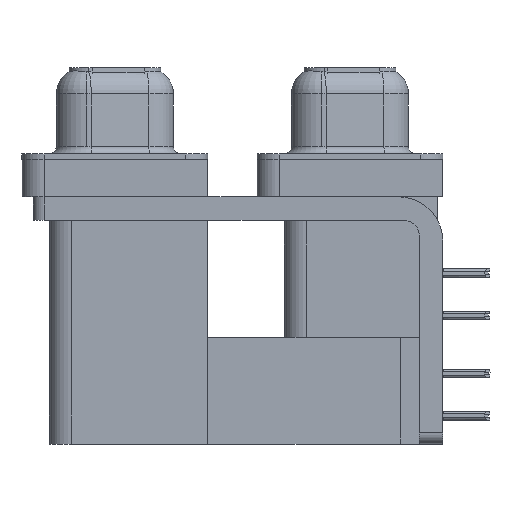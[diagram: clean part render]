
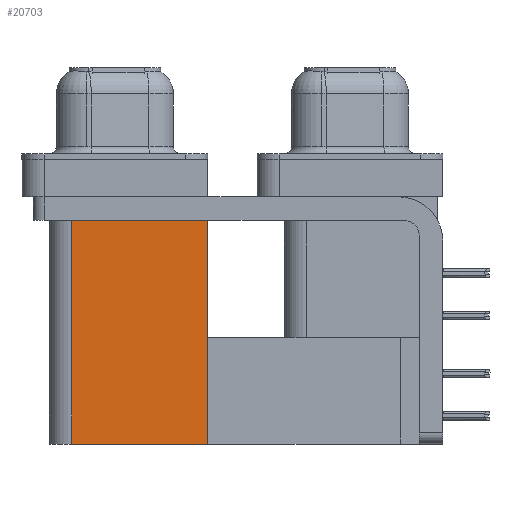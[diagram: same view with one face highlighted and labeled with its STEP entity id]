
A CAD part, left-side view. The second image highlights one B-rep face of the part: STEP entity #20703.
In plain terms, the highlighted planar face has unit normal (-1, 0, 0).
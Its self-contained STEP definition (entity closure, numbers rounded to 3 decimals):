
#414 = EDGE_LOOP ( 'NONE', ( #9006, #5287, #41787, #28909 ) ) ;
#511 = DIRECTION ( 'NONE',  ( 1., 0., 0. ) ) ;
#982 = CARTESIAN_POINT ( 'NONE',  ( 3.765, 9.6, -19.2 ) ) ;
#1129 = CARTESIAN_POINT ( 'NONE',  ( 3.765, 18.8, -19.2 ) ) ;
#2963 = CARTESIAN_POINT ( 'NONE',  ( 3.765, 18.8, -2.5 ) ) ;
#3436 = VECTOR ( 'NONE', #10936, 1000. ) ;
#5287 = ORIENTED_EDGE ( 'NONE', *, *, #42989, .F. ) ;
#5908 = VECTOR ( 'NONE', #14728, 1000. ) ;
#6147 = VERTEX_POINT ( 'NONE', #2963 ) ;
#6846 = PLANE ( 'NONE',  #42145 ) ;
#7087 = CARTESIAN_POINT ( 'NONE',  ( 3.765, 9.6, -19.2 ) ) ;
#7675 = CARTESIAN_POINT ( 'NONE',  ( 3.765, 9.6, -19.2 ) ) ;
#9006 = ORIENTED_EDGE ( 'NONE', *, *, #37105, .T. ) ;
#10936 = DIRECTION ( 'NONE',  ( 0., 1., 0. ) ) ;
#14728 = DIRECTION ( 'NONE',  ( 0., 0., 1. ) ) ;
#19358 = CARTESIAN_POINT ( 'NONE',  ( 3.765, 9.6, -19.2 ) ) ;
#19516 = DIRECTION ( 'NONE',  ( 0., 1., 0. ) ) ;
#20703 = ADVANCED_FACE ( 'NONE', ( #38991 ), #6846, .F. ) ;
#20793 = CARTESIAN_POINT ( 'NONE',  ( 3.765, 18.8, -19.2 ) ) ;
#21824 = CARTESIAN_POINT ( 'NONE',  ( 3.765, 9.6, -2.5 ) ) ;
#24299 = LINE ( 'NONE', #20793, #43199 ) ;
#25811 = VERTEX_POINT ( 'NONE', #1129 ) ;
#28909 = ORIENTED_EDGE ( 'NONE', *, *, #45915, .T. ) ;
#32282 = CARTESIAN_POINT ( 'NONE',  ( 3.765, 9.6, -2.5 ) ) ;
#33144 = VERTEX_POINT ( 'NONE', #19358 ) ;
#35090 = DIRECTION ( 'NONE',  ( 0., 0., 1. ) ) ;
#37105 = EDGE_CURVE ( 'NONE', #44500, #6147, #45663, .T. ) ;
#38991 = FACE_OUTER_BOUND ( 'NONE', #414, .T. ) ;
#41787 = ORIENTED_EDGE ( 'NONE', *, *, #44243, .F. ) ;
#42145 = AXIS2_PLACEMENT_3D ( 'NONE', #7087, #511, #42979 ) ;
#42979 = DIRECTION ( 'NONE',  ( 0., 0., -1. ) ) ;
#42989 = EDGE_CURVE ( 'NONE', #25811, #6147, #24299, .T. ) ;
#43199 = VECTOR ( 'NONE', #35090, 1000. ) ;
#44243 = EDGE_CURVE ( 'NONE', #33144, #25811, #44363, .T. ) ;
#44363 = LINE ( 'NONE', #982, #46251 ) ;
#44500 = VERTEX_POINT ( 'NONE', #21824 ) ;
#45663 = LINE ( 'NONE', #32282, #3436 ) ;
#45915 = EDGE_CURVE ( 'NONE', #33144, #44500, #46165, .T. ) ;
#46165 = LINE ( 'NONE', #7675, #5908 ) ;
#46251 = VECTOR ( 'NONE', #19516, 1000. ) ;
